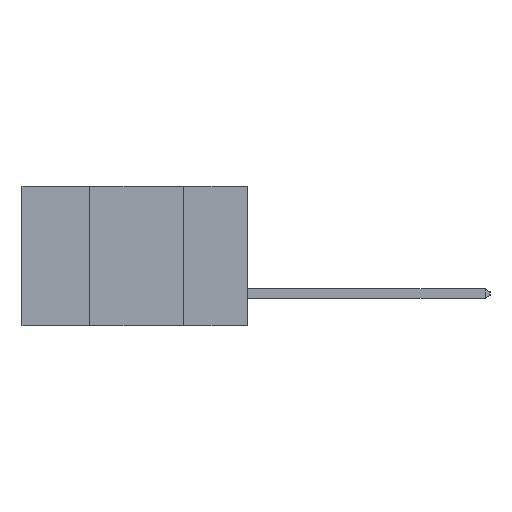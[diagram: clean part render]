
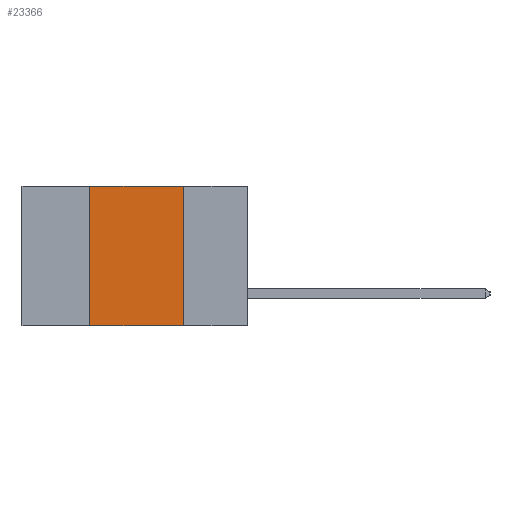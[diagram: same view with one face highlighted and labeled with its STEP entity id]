
A CAD part, left-side view. The second image highlights one B-rep face of the part: STEP entity #23366.
In plain terms, the highlighted planar face has unit normal (-1, 0, 0).
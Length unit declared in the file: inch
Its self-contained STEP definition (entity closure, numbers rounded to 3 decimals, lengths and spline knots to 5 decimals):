
#90 = DIRECTION ( 'NONE',  ( 0., -1., 0. ) ) ;
#105 = DIRECTION ( 'NONE',  ( 0., -1., 0. ) ) ;
#244 = CARTESIAN_POINT ( 'NONE',  ( 0., 0.6, -0.37 ) ) ;
#993 = ORIENTED_EDGE ( 'NONE', *, *, #12294, .F. ) ;
#1399 = VERTEX_POINT ( 'NONE', #12296 ) ;
#2122 = VECTOR ( 'NONE', #90, 39.37008 ) ;
#2983 = FACE_OUTER_BOUND ( 'NONE', #5922, .T. ) ;
#3235 = DIRECTION ( 'NONE',  ( 0., 0., 1. ) ) ;
#3314 = VECTOR ( 'NONE', #105, 39.37008 ) ;
#3577 = ORIENTED_EDGE ( 'NONE', *, *, #14620, .F. ) ;
#4612 = EDGE_CURVE ( 'NONE', #1399, #8013, #14021, .T. ) ;
#4793 = EDGE_CURVE ( 'NONE', #6625, #8013, #14313, .T. ) ;
#5356 = DIRECTION ( 'NONE',  ( 1., 0., 0. ) ) ;
#5922 = EDGE_LOOP ( 'NONE', ( #15845, #993, #3577, #9260 ) ) ;
#6625 = VERTEX_POINT ( 'NONE', #12319 ) ;
#7947 = CARTESIAN_POINT ( 'NONE',  ( 0., 0.42, 0. ) ) ;
#8013 = VERTEX_POINT ( 'NONE', #24081 ) ;
#9260 = ORIENTED_EDGE ( 'NONE', *, *, #4612, .T. ) ;
#12294 = EDGE_CURVE ( 'NONE', #19707, #6625, #15369, .T. ) ;
#12296 = CARTESIAN_POINT ( 'NONE',  ( 0., 0.42, -0.37 ) ) ;
#12319 = CARTESIAN_POINT ( 'NONE',  ( 0., 0.17, 0. ) ) ;
#12667 = CARTESIAN_POINT ( 'NONE',  ( 0., 0.6, 0. ) ) ;
#13382 = CARTESIAN_POINT ( 'NONE',  ( 0., 0.6, 0. ) ) ;
#13702 = VECTOR ( 'NONE', #16001, 39.37008 ) ;
#14021 = LINE ( 'NONE', #244, #3314 ) ;
#14313 = LINE ( 'NONE', #17136, #13702 ) ;
#14620 = EDGE_CURVE ( 'NONE', #1399, #19707, #24586, .T. ) ;
#15369 = LINE ( 'NONE', #12667, #2122 ) ;
#15845 = ORIENTED_EDGE ( 'NONE', *, *, #4793, .F. ) ;
#16001 = DIRECTION ( 'NONE',  ( 0., 0., -1. ) ) ;
#16069 = AXIS2_PLACEMENT_3D ( 'NONE', #13382, #5356, #19185 ) ;
#17136 = CARTESIAN_POINT ( 'NONE',  ( 0., 0.17, -0.37 ) ) ;
#17296 = PLANE ( 'NONE',  #16069 ) ;
#19185 = DIRECTION ( 'NONE',  ( 0., 0., -1. ) ) ;
#19669 = VECTOR ( 'NONE', #3235, 39.37008 ) ;
#19707 = VERTEX_POINT ( 'NONE', #7947 ) ;
#23366 = ADVANCED_FACE ( 'NONE', ( #2983 ), #17296, .F. ) ;
#24081 = CARTESIAN_POINT ( 'NONE',  ( 0., 0.17, -0.37 ) ) ;
#24586 = LINE ( 'NONE', #24595, #19669 ) ;
#24595 = CARTESIAN_POINT ( 'NONE',  ( 0., 0.42, -0.37 ) ) ;
